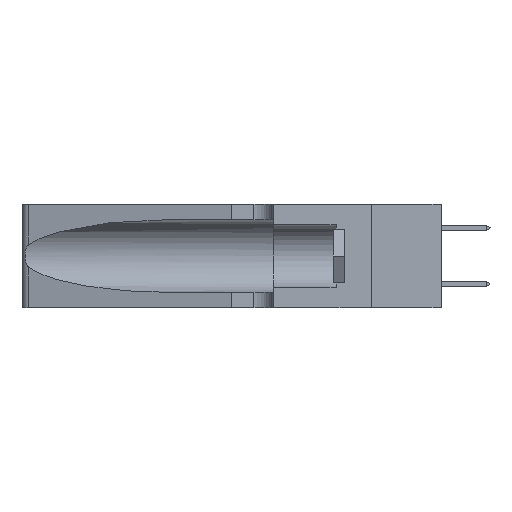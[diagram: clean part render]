
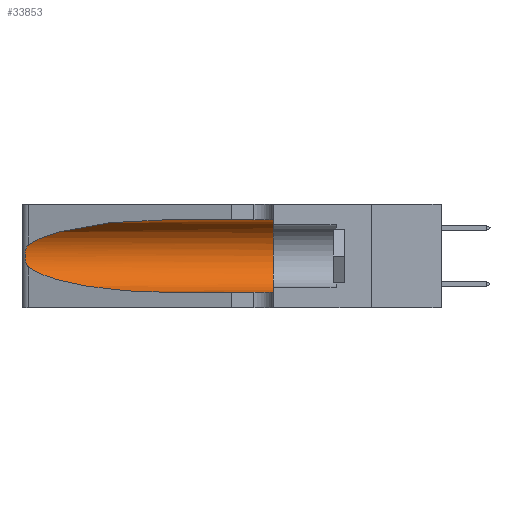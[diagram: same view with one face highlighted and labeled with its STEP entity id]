
A CAD part, left-side view. The second image highlights one B-rep face of the part: STEP entity #33853.
In plain terms, the highlighted cylindrical face has radius 3.308 mm (diameter 6.617 mm), a partial arc.
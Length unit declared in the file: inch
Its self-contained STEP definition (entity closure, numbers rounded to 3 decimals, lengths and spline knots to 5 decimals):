
#15 = CARTESIAN_POINT ( 'NONE',  ( 0.1305, 0.72297, 0.31525 ) ) ;
#601 = AXIS2_PLACEMENT_3D ( 'NONE', #6378, #33011, #976 ) ;
#883 = AXIS2_PLACEMENT_3D ( 'NONE', #6739, #8953, #33123 ) ;
#976 = DIRECTION ( 'NONE',  ( 0., 0., -1. ) ) ;
#1602 = CARTESIAN_POINT ( 'NONE',  ( 0.25856, 1.23593, 0.16098 ) ) ;
#1950 = FACE_OUTER_BOUND ( 'NONE', #8397, .T. ) ;
#1982 = CARTESIAN_POINT ( 'NONE',  ( 0.18966, 0.96281, 0.31525 ) ) ;
#2915 =( BOUNDED_CURVE ( )  B_SPLINE_CURVE ( 3, ( #17977, #1982, #26667, #32871 ),
 .UNSPECIFIED., .F., .T. ) 
 B_SPLINE_CURVE_WITH_KNOTS ( ( 4, 4 ),
 ( 1.5708, 2.84003 ),
 .UNSPECIFIED. ) 
 CURVE ( )  GEOMETRIC_REPRESENTATION_ITEM ( )  RATIONAL_B_SPLINE_CURVE ( ( 1., 0.87, 0.87, 1. ) ) 
 REPRESENTATION_ITEM ( '' )  );
#2962 = VERTEX_POINT ( 'NONE', #5552 ) ;
#4208 = CARTESIAN_POINT ( 'NONE',  ( 0.25787, 1.23484, 0.2124 ) ) ;
#4329 = CARTESIAN_POINT ( 'NONE',  ( 0.25789, 1.23486, 0.15765 ) ) ;
#5429 = CIRCLE ( 'NONE', #883, 0.13025 ) ;
#5552 = CARTESIAN_POINT ( 'NONE',  ( 0.1305, 0.72297, 0.05475 ) ) ;
#6378 = CARTESIAN_POINT ( 'NONE',  ( 0.1305, 1.61858, 0.185 ) ) ;
#6739 = CARTESIAN_POINT ( 'NONE',  ( 0.1305, 0.35, 0.185 ) ) ;
#7096 = VERTEX_POINT ( 'NONE', #22695 ) ;
#7285 = EDGE_CURVE ( 'NONE', #2962, #14261, #27243, .T. ) ;
#7657 = B_SPLINE_CURVE_WITH_KNOTS ( 'NONE', 3,
 ( #11632, #25616, #20210, #4208, #9580, #14594, #12256, #33624, #17642, #1602, #4329, #23056, #30499, #11872 ),
 .UNSPECIFIED., .F., .F.,
 ( 4, 2, 2, 2, 2, 2, 4 ),
 ( 0., 0.00027, 0.00053, 0.00107, 0.0016, 0.00187, 0.00214 ),
 .UNSPECIFIED. ) ;
#7681 = EDGE_CURVE ( 'NONE', #31888, #15683, #9629, .T. ) ;
#7822 = EDGE_CURVE ( 'NONE', #15683, #14261, #5429, .T. ) ;
#8397 = EDGE_LOOP ( 'NONE', ( #19168, #27805, #31432, #14525, #28634, #13638 ) ) ;
#8953 = DIRECTION ( 'NONE',  ( 0., 1., 0. ) ) ;
#9076 =( BOUNDED_CURVE ( )  B_SPLINE_CURVE ( 3, ( #26736, #10700, #15856, #23975 ),
 .UNSPECIFIED., .F., .F. ) 
 B_SPLINE_CURVE_WITH_KNOTS ( ( 4, 4 ),
 ( 3.44316, 4.71239 ),
 .UNSPECIFIED. ) 
 CURVE ( )  GEOMETRIC_REPRESENTATION_ITEM ( )  RATIONAL_B_SPLINE_CURVE ( ( 1., 0.87, 0.87, 1. ) ) 
 REPRESENTATION_ITEM ( '' )  );
#9580 = CARTESIAN_POINT ( 'NONE',  ( 0.25854, 1.2359, 0.20912 ) ) ;
#9629 = LINE ( 'NONE', #11089, #24709 ) ;
#10700 = CARTESIAN_POINT ( 'NONE',  ( 0.2373, 1.15595, 0.08982 ) ) ;
#11089 = CARTESIAN_POINT ( 'NONE',  ( 0.1305, 1.61858, 0.31525 ) ) ;
#11297 = VECTOR ( 'NONE', #25528, 39.37008 ) ;
#11632 = CARTESIAN_POINT ( 'NONE',  ( 0.25487, 1.22718, 0.22369 ) ) ;
#11872 = CARTESIAN_POINT ( 'NONE',  ( 0.25487, 1.22718, 0.14631 ) ) ;
#12256 = CARTESIAN_POINT ( 'NONE',  ( 0.26075, 1.23896, 0.19203 ) ) ;
#12826 = CYLINDRICAL_SURFACE ( 'NONE', #601, 0.13025 ) ;
#13411 = VERTEX_POINT ( 'NONE', #30867 ) ;
#13638 = ORIENTED_EDGE ( 'NONE', *, *, #7681, .F. ) ;
#14261 = VERTEX_POINT ( 'NONE', #30259 ) ;
#14525 = ORIENTED_EDGE ( 'NONE', *, *, #7285, .T. ) ;
#14594 = CARTESIAN_POINT ( 'NONE',  ( 0.26018, 1.23835, 0.19895 ) ) ;
#15683 = VERTEX_POINT ( 'NONE', #18057 ) ;
#15856 = CARTESIAN_POINT ( 'NONE',  ( 0.18966, 0.96281, 0.05475 ) ) ;
#17642 = CARTESIAN_POINT ( 'NONE',  ( 0.26017, 1.23833, 0.17102 ) ) ;
#17977 = CARTESIAN_POINT ( 'NONE',  ( 0.1305, 0.72297, 0.31525 ) ) ;
#18057 = CARTESIAN_POINT ( 'NONE',  ( 0.1305, 0.35, 0.31525 ) ) ;
#19168 = ORIENTED_EDGE ( 'NONE', *, *, #23998, .T. ) ;
#20210 = CARTESIAN_POINT ( 'NONE',  ( 0.25639, 1.23184, 0.21858 ) ) ;
#20961 = EDGE_CURVE ( 'NONE', #7096, #13411, #7657, .T. ) ;
#22695 = CARTESIAN_POINT ( 'NONE',  ( 0.25487, 1.22718, 0.22369 ) ) ;
#22750 = EDGE_CURVE ( 'NONE', #13411, #2962, #9076, .T. ) ;
#22966 = CARTESIAN_POINT ( 'NONE',  ( 0.1305, 1.61858, 0.05475 ) ) ;
#23056 = CARTESIAN_POINT ( 'NONE',  ( 0.25639, 1.23186, 0.15144 ) ) ;
#23975 = CARTESIAN_POINT ( 'NONE',  ( 0.1305, 0.72297, 0.05475 ) ) ;
#23998 = EDGE_CURVE ( 'NONE', #31888, #7096, #2915, .T. ) ;
#24709 = VECTOR ( 'NONE', #34310, 39.37008 ) ;
#25528 = DIRECTION ( 'NONE',  ( 0., -1., 0. ) ) ;
#25616 = CARTESIAN_POINT ( 'NONE',  ( 0.25555, 1.22994, 0.2215 ) ) ;
#26667 = CARTESIAN_POINT ( 'NONE',  ( 0.2373, 1.15595, 0.28018 ) ) ;
#26736 = CARTESIAN_POINT ( 'NONE',  ( 0.25487, 1.22718, 0.14631 ) ) ;
#27243 = LINE ( 'NONE', #22966, #11297 ) ;
#27805 = ORIENTED_EDGE ( 'NONE', *, *, #20961, .T. ) ;
#28634 = ORIENTED_EDGE ( 'NONE', *, *, #7822, .F. ) ;
#30259 = CARTESIAN_POINT ( 'NONE',  ( 0.1305, 0.35, 0.05475 ) ) ;
#30499 = CARTESIAN_POINT ( 'NONE',  ( 0.25555, 1.22993, 0.14849 ) ) ;
#30867 = CARTESIAN_POINT ( 'NONE',  ( 0.25487, 1.22718, 0.14631 ) ) ;
#31432 = ORIENTED_EDGE ( 'NONE', *, *, #22750, .T. ) ;
#31888 = VERTEX_POINT ( 'NONE', #15 ) ;
#32871 = CARTESIAN_POINT ( 'NONE',  ( 0.25487, 1.22718, 0.22369 ) ) ;
#33011 = DIRECTION ( 'NONE',  ( 0., -1., 0. ) ) ;
#33123 = DIRECTION ( 'NONE',  ( 0., 0., 1. ) ) ;
#33624 = CARTESIAN_POINT ( 'NONE',  ( 0.26075, 1.23896, 0.178 ) ) ;
#33853 = ADVANCED_FACE ( 'NONE', ( #1950 ), #12826, .F. ) ;
#34310 = DIRECTION ( 'NONE',  ( 0., -1., 0. ) ) ;
